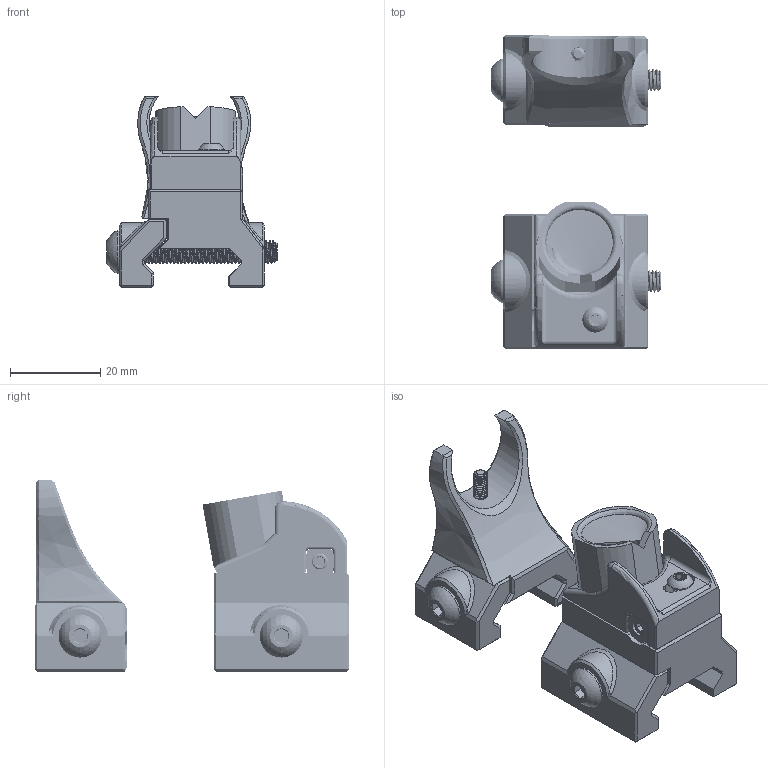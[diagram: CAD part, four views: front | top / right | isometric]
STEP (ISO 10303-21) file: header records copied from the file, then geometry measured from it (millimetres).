
FILE_DESCRIPTION(/* description */ (''),/* implementation_level */ '2;1');
FILE_NAME(/* name */ 'Picatinny Diopter Sights v1.step',/* time_stamp */ '2022-08-07T23:14:11-04:00',/* author */ (''),/* organization */ (''),/* preprocessor_version */ 'ST-DEVELOPER v19',/* originating_system */ 'Autodesk Translation Framework v11.7.0.108',/* authorisation */ '');
FILE_SCHEMA (('AUTOMOTIVE_DESIGN { 1 0 10303 214 3 1 1 }'));
Products named in the file (21): Picatinny Diopter Sights v1; Rear Sight; Hardware; M3 Threaded Insert (1)^X Carriage Frame_X Carriage; M3 Threaded Insert (1)^X Carriage Frame_X Carriage (2); M3x8 SHCS or BHCS 91290A113_Alloy Steel Socket Head Screw; M3x10 BHCS 91239A113_Button Head Hex Drive Screw; 3mm Washer 94744A711_Zinc-Plated Steel Washer for Soft Material; M3 Threaded Insert (1)^X Carriage Frame_X Carriage (3); M3x15 BHCS 91239A811_Button Head Hex Drive Screw; Drum Slide; Drum; Rear Sight Base; M5 Hex Nut 90593A004_Black-Oxide Steel Hex Nut; M5x35 BHCS 91239A238_Button Head Hex Drive Screw (1); Front Sight; Hardware (1); M3x20 SHCS 91274A109_Zinc-Aluminum-Coated Alloy Steel Socket Head Scr
ew; M3 Threaded Insert (1)^X Carriage Frame_X Carriage (1); M5 Nut 90593A004_Black-Oxide Steel Hex Nut (1); M5x35 BHCS 91239A238_Button Head Hex Drive Screw
Assembly tree (21 placements, depth 4):
  Picatinny Diopter Sights v1
    Rear Sight
      Hardware
        M3 Threaded Insert (1)^X Carriage Frame_X Carriage
        M3 Threaded Insert (1)^X Carriage Frame_X Carriage (2)
        M3x8 SHCS or BHCS 91290A113_Alloy Steel Socket Head Screw
        M3x10 BHCS 91239A113_Button Head Hex Drive Screw
        3mm Washer 94744A711_Zinc-Plated Steel Washer for Soft Material  x2
        M3 Threaded Insert (1)^X Carriage Frame_X Carriage (3)
        M3x15 BHCS 91239A811_Button Head Hex Drive Screw
      Drum Slide
      Drum
      Rear Sight Base
        M5 Hex Nut 90593A004_Black-Oxide Steel Hex Nut
        M5x35 BHCS 91239A238_Button Head Hex Drive Screw (1)
    Front Sight
      Hardware (1)
        M3x20 SHCS 91274A109_Zinc-Aluminum-Coated Alloy Steel Socket Head Scr
ew
        M3 Threaded Insert (1)^X Carriage Frame_X Carriage (1)
        M5 Nut 90593A004_Black-Oxide Steel Hex Nut (1)
        M5x35 BHCS 91239A238_Button Head Hex Drive Screw
Bounding box: 37.78 x 69.6 x 42.5 mm (x, y, z)
Volume: 29165.8 mm3; surface area: 19434.9 mm2
Topology: 21 solids, 21 shells, 1842 faces, 4749 edges, 3075 vertices
Faces by surface type: plane 742, cylinder 604, bspline 356, cone 116, torus 18, sphere 6
Full cylindrical faces by diameter (mm): 1.5 x3, 2 x1, 2.35 x92, 2.9 x4, 3 x96, 3.1 x5, 3.2 x1, 3.5 x2, 3.961 x88, 4.2 x10, 4.25 x4, 4.6 x4, 5 x96, 5.5 x2, 5.6 x1, 5.7 x2, 6.8 x2, 8 x1, 8.2 x1, 9.5 x2
Entity records: 112825 total; most frequent: CARTESIAN_POINT 70556, ORIENTED_EDGE 9482, DIRECTION 7434, EDGE_CURVE 4741, VERTEX_POINT 3071, AXIS2_PLACEMENT_3D 2759, EDGE_LOOP 2008, LINE 1916
